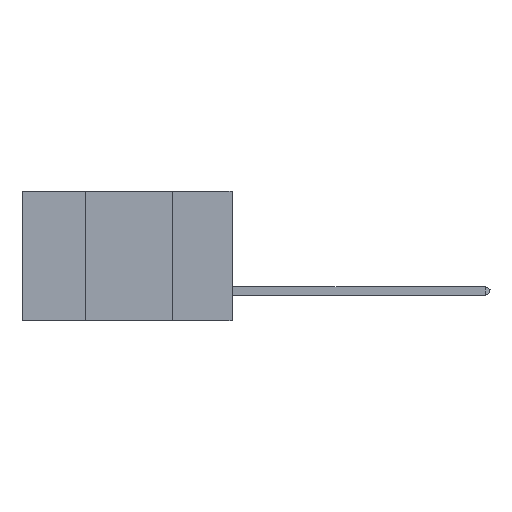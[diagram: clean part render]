
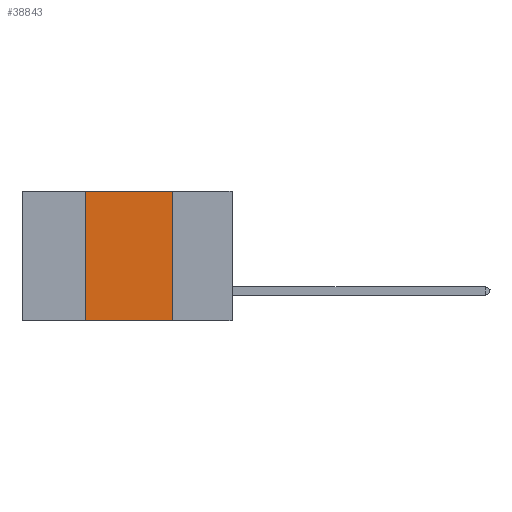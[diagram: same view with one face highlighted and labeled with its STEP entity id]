
A CAD part, left-side view. The second image highlights one B-rep face of the part: STEP entity #38843.
In plain terms, the highlighted planar face has unit normal (-1, 0, 0).
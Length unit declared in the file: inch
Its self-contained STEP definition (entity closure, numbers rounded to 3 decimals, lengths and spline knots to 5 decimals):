
#2065 = EDGE_CURVE ( 'NONE', #27765, #27516, #33416, .T. ) ;
#2152 = CARTESIAN_POINT ( 'NONE',  ( 0., 0.6, 0. ) ) ;
#2748 = LINE ( 'NONE', #2152, #10866 ) ;
#7910 = DIRECTION ( 'NONE',  ( 1., 0., 0. ) ) ;
#9288 = LINE ( 'NONE', #21485, #16388 ) ;
#10202 = VERTEX_POINT ( 'NONE', #19547 ) ;
#10226 = EDGE_LOOP ( 'NONE', ( #15650, #38385, #37193, #26993 ) ) ;
#10817 = EDGE_CURVE ( 'NONE', #27765, #10202, #38543, .T. ) ;
#10866 = VECTOR ( 'NONE', #38755, 39.37008 ) ;
#13464 = CARTESIAN_POINT ( 'NONE',  ( 0., 0.42, 0. ) ) ;
#13868 = PLANE ( 'NONE',  #34808 ) ;
#13972 = CARTESIAN_POINT ( 'NONE',  ( 0., 0.42, 0. ) ) ;
#15650 = ORIENTED_EDGE ( 'NONE', *, *, #38267, .F. ) ;
#16388 = VECTOR ( 'NONE', #24576, 39.37008 ) ;
#16551 = DIRECTION ( 'NONE',  ( 0., 0., 1. ) ) ;
#19181 = CARTESIAN_POINT ( 'NONE',  ( 0., 0.17, 0. ) ) ;
#19547 = CARTESIAN_POINT ( 'NONE',  ( 0., 0.17, -0.37 ) ) ;
#20308 = CARTESIAN_POINT ( 'NONE',  ( 0., 0.6, 0. ) ) ;
#21485 = CARTESIAN_POINT ( 'NONE',  ( 0., 0.17, 0. ) ) ;
#22656 = FACE_OUTER_BOUND ( 'NONE', #10226, .T. ) ;
#22888 = EDGE_CURVE ( 'NONE', #27516, #36596, #2748, .T. ) ;
#24004 = CARTESIAN_POINT ( 'NONE',  ( 0., 0.42, -0.37 ) ) ;
#24112 = DIRECTION ( 'NONE',  ( 0., 0., -1. ) ) ;
#24576 = DIRECTION ( 'NONE',  ( 0., 0., -1. ) ) ;
#26993 = ORIENTED_EDGE ( 'NONE', *, *, #10817, .T. ) ;
#27516 = VERTEX_POINT ( 'NONE', #13972 ) ;
#27765 = VERTEX_POINT ( 'NONE', #24004 ) ;
#27773 = DIRECTION ( 'NONE',  ( 0., -1., 0. ) ) ;
#33416 = LINE ( 'NONE', #13464, #34801 ) ;
#34801 = VECTOR ( 'NONE', #16551, 39.37008 ) ;
#34808 = AXIS2_PLACEMENT_3D ( 'NONE', #20308, #7910, #24112 ) ;
#36596 = VERTEX_POINT ( 'NONE', #19181 ) ;
#37068 = VECTOR ( 'NONE', #27773, 39.37008 ) ;
#37193 = ORIENTED_EDGE ( 'NONE', *, *, #2065, .F. ) ;
#38267 = EDGE_CURVE ( 'NONE', #36596, #10202, #9288, .T. ) ;
#38385 = ORIENTED_EDGE ( 'NONE', *, *, #22888, .F. ) ;
#38543 = LINE ( 'NONE', #39170, #37068 ) ;
#38755 = DIRECTION ( 'NONE',  ( 0., -1., 0. ) ) ;
#38843 = ADVANCED_FACE ( 'NONE', ( #22656 ), #13868, .F. ) ;
#39170 = CARTESIAN_POINT ( 'NONE',  ( 0., 0.6, -0.37 ) ) ;
